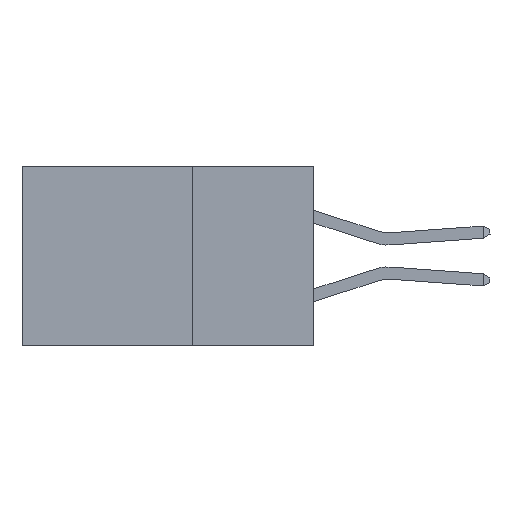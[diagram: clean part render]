
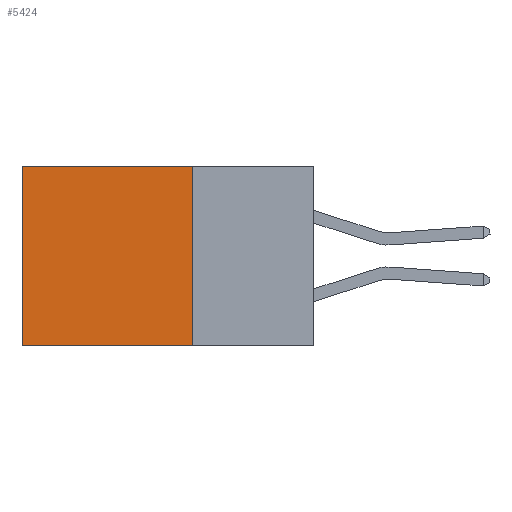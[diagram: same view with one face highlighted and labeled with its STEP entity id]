
A CAD part, left-side view. The second image highlights one B-rep face of the part: STEP entity #5424.
In plain terms, the highlighted planar face has unit normal (-1, 0, 0).
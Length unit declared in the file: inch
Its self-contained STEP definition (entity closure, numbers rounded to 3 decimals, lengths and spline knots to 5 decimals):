
#451 = EDGE_CURVE ( 'NONE', #2435, #13575, #11409, .T. ) ;
#731 = EDGE_CURVE ( 'NONE', #12084, #13575, #1865, .T. ) ;
#758 = DIRECTION ( 'NONE',  ( 0., 0., -1. ) ) ;
#1117 = VECTOR ( 'NONE', #12586, 39.37008 ) ;
#1135 = VERTEX_POINT ( 'NONE', #6212 ) ;
#1238 = AXIS2_PLACEMENT_3D ( 'NONE', #13924, #9624, #14001 ) ;
#1256 = CARTESIAN_POINT ( 'NONE',  ( 0.2875, 0.25, 0. ) ) ;
#1414 = CARTESIAN_POINT ( 'NONE',  ( 0.2875, 0.25, 0. ) ) ;
#1865 = LINE ( 'NONE', #6368, #2112 ) ;
#2112 = VECTOR ( 'NONE', #758, 39.37008 ) ;
#2435 = VERTEX_POINT ( 'NONE', #5053 ) ;
#3023 = VECTOR ( 'NONE', #9242, 39.37008 ) ;
#4119 = CARTESIAN_POINT ( 'NONE',  ( 0.2875, 0.6, 0. ) ) ;
#5019 = EDGE_LOOP ( 'NONE', ( #14456, #5155, #7782, #6455 ) ) ;
#5053 = CARTESIAN_POINT ( 'NONE',  ( 0.2875, 0.25, -0.37 ) ) ;
#5155 = ORIENTED_EDGE ( 'NONE', *, *, #451, .F. ) ;
#5424 = ADVANCED_FACE ( 'NONE', ( #11913 ), #9694, .F. ) ;
#5979 = LINE ( 'NONE', #1256, #3023 ) ;
#6212 = CARTESIAN_POINT ( 'NONE',  ( 0.2875, 0.25, 0. ) ) ;
#6368 = CARTESIAN_POINT ( 'NONE',  ( 0.2875, 0.6, 0. ) ) ;
#6455 = ORIENTED_EDGE ( 'NONE', *, *, #8875, .T. ) ;
#7735 = CARTESIAN_POINT ( 'NONE',  ( 0.2875, 0.25, -0.37 ) ) ;
#7782 = ORIENTED_EDGE ( 'NONE', *, *, #8465, .F. ) ;
#8465 = EDGE_CURVE ( 'NONE', #1135, #2435, #13857, .T. ) ;
#8875 = EDGE_CURVE ( 'NONE', #1135, #12084, #5979, .T. ) ;
#9242 = DIRECTION ( 'NONE',  ( 0., 1., 0. ) ) ;
#9624 = DIRECTION ( 'NONE',  ( 1., 0., 0. ) ) ;
#9694 = PLANE ( 'NONE',  #1238 ) ;
#9874 = CARTESIAN_POINT ( 'NONE',  ( 0.2875, 0.6, -0.37 ) ) ;
#11409 = LINE ( 'NONE', #7735, #11563 ) ;
#11563 = VECTOR ( 'NONE', #12242, 39.37008 ) ;
#11913 = FACE_OUTER_BOUND ( 'NONE', #5019, .T. ) ;
#12084 = VERTEX_POINT ( 'NONE', #4119 ) ;
#12242 = DIRECTION ( 'NONE',  ( 0., 1., 0. ) ) ;
#12586 = DIRECTION ( 'NONE',  ( 0., 0., -1. ) ) ;
#13575 = VERTEX_POINT ( 'NONE', #9874 ) ;
#13857 = LINE ( 'NONE', #1414, #1117 ) ;
#13924 = CARTESIAN_POINT ( 'NONE',  ( 0.2875, 0.25, 0. ) ) ;
#14001 = DIRECTION ( 'NONE',  ( 0., 0., -1. ) ) ;
#14456 = ORIENTED_EDGE ( 'NONE', *, *, #731, .T. ) ;
